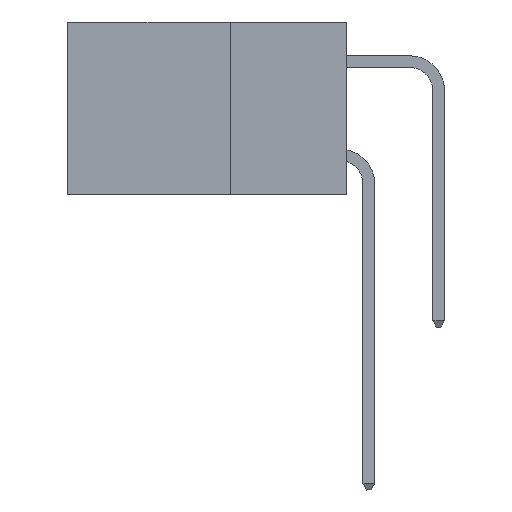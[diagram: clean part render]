
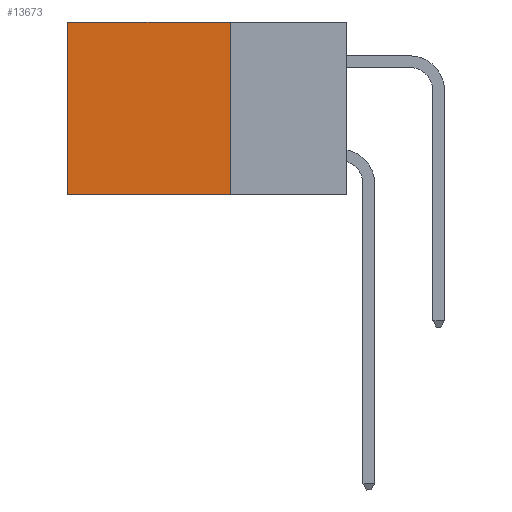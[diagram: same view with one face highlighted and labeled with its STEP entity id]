
A CAD part, left-side view. The second image highlights one B-rep face of the part: STEP entity #13673.
In plain terms, the highlighted planar face has unit normal (-1, 0, 0).
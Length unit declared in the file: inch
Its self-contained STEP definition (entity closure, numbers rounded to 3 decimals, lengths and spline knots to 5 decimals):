
#120 = EDGE_CURVE ( 'NONE', #10081, #9003, #6578, .T. ) ;
#386 = DIRECTION ( 'NONE',  ( 0., 0., -1. ) ) ;
#439 = CARTESIAN_POINT ( 'NONE',  ( 0.2875, 0.6, 0. ) ) ;
#781 = AXIS2_PLACEMENT_3D ( 'NONE', #7022, #8839, #21569 ) ;
#790 = FACE_OUTER_BOUND ( 'NONE', #19384, .T. ) ;
#819 = ORIENTED_EDGE ( 'NONE', *, *, #120, .T. ) ;
#2878 = DIRECTION ( 'NONE',  ( 0., 1., 0. ) ) ;
#4391 = EDGE_CURVE ( 'NONE', #9482, #9003, #18715, .T. ) ;
#5221 = PLANE ( 'NONE',  #781 ) ;
#5510 = VECTOR ( 'NONE', #2878, 39.37008 ) ;
#6578 = LINE ( 'NONE', #16698, #21088 ) ;
#7022 = CARTESIAN_POINT ( 'NONE',  ( 0.2875, 0.25, 0. ) ) ;
#8839 = DIRECTION ( 'NONE',  ( 1., 0., 0. ) ) ;
#9003 = VERTEX_POINT ( 'NONE', #20252 ) ;
#9116 = DIRECTION ( 'NONE',  ( 0., 0., -1. ) ) ;
#9482 = VERTEX_POINT ( 'NONE', #12761 ) ;
#9977 = LINE ( 'NONE', #11167, #19670 ) ;
#10081 = VERTEX_POINT ( 'NONE', #439 ) ;
#10928 = ORIENTED_EDGE ( 'NONE', *, *, #4391, .F. ) ;
#10981 = CARTESIAN_POINT ( 'NONE',  ( 0.2875, 0.25, 0. ) ) ;
#11167 = CARTESIAN_POINT ( 'NONE',  ( 0.2875, 0.25, 0. ) ) ;
#12761 = CARTESIAN_POINT ( 'NONE',  ( 0.2875, 0.25, -0.37 ) ) ;
#13673 = ADVANCED_FACE ( 'NONE', ( #790 ), #5221, .F. ) ;
#13870 = VECTOR ( 'NONE', #22008, 39.37008 ) ;
#14091 = EDGE_CURVE ( 'NONE', #19637, #10081, #19439, .T. ) ;
#14290 = ORIENTED_EDGE ( 'NONE', *, *, #14091, .T. ) ;
#15172 = EDGE_CURVE ( 'NONE', #19637, #9482, #9977, .T. ) ;
#16698 = CARTESIAN_POINT ( 'NONE',  ( 0.2875, 0.6, 0. ) ) ;
#18387 = CARTESIAN_POINT ( 'NONE',  ( 0.2875, 0.25, -0.37 ) ) ;
#18715 = LINE ( 'NONE', #18387, #13870 ) ;
#19168 = CARTESIAN_POINT ( 'NONE',  ( 0.2875, 0.25, 0. ) ) ;
#19384 = EDGE_LOOP ( 'NONE', ( #819, #10928, #19485, #14290 ) ) ;
#19439 = LINE ( 'NONE', #19168, #5510 ) ;
#19485 = ORIENTED_EDGE ( 'NONE', *, *, #15172, .F. ) ;
#19637 = VERTEX_POINT ( 'NONE', #10981 ) ;
#19670 = VECTOR ( 'NONE', #386, 39.37008 ) ;
#20252 = CARTESIAN_POINT ( 'NONE',  ( 0.2875, 0.6, -0.37 ) ) ;
#21088 = VECTOR ( 'NONE', #9116, 39.37008 ) ;
#21569 = DIRECTION ( 'NONE',  ( 0., 0., -1. ) ) ;
#22008 = DIRECTION ( 'NONE',  ( 0., 1., 0. ) ) ;
